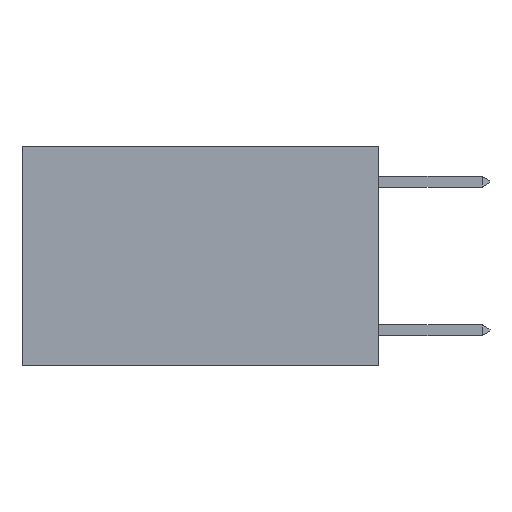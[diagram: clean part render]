
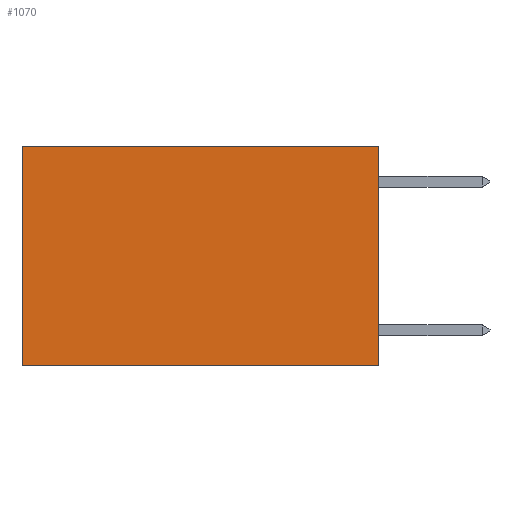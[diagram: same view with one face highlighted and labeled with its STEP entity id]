
A CAD part, left-side view. The second image highlights one B-rep face of the part: STEP entity #1070.
In plain terms, the highlighted planar face has unit normal (-1, 0, 0).
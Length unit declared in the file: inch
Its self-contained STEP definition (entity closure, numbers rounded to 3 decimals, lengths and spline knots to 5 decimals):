
#16 = VECTOR ( 'NONE', #1079, 39.37008 ) ;
#776 = AXIS2_PLACEMENT_3D ( 'NONE', #7842, #1541, #2116 ) ;
#898 = VERTEX_POINT ( 'NONE', #2107 ) ;
#1070 = ADVANCED_FACE ( 'NONE', ( #6622 ), #2194, .F. ) ;
#1079 = DIRECTION ( 'NONE',  ( 0., 1., 0. ) ) ;
#1117 = CARTESIAN_POINT ( 'NONE',  ( 0.2625, 0., 0. ) ) ;
#1541 = DIRECTION ( 'NONE',  ( 1., 0., 0. ) ) ;
#1621 = VERTEX_POINT ( 'NONE', #4800 ) ;
#1690 = VECTOR ( 'NONE', #4601, 39.37008 ) ;
#1726 = VECTOR ( 'NONE', #1788, 39.37008 ) ;
#1788 = DIRECTION ( 'NONE',  ( 0., 1., 0. ) ) ;
#2107 = CARTESIAN_POINT ( 'NONE',  ( 0.2625, 0., -0.37 ) ) ;
#2116 = DIRECTION ( 'NONE',  ( 0., 0., -1. ) ) ;
#2120 = LINE ( 'NONE', #5895, #4233 ) ;
#2194 = PLANE ( 'NONE',  #776 ) ;
#2446 = LINE ( 'NONE', #1117, #1690 ) ;
#2507 = DIRECTION ( 'NONE',  ( 0., 0., -1. ) ) ;
#2622 = ORIENTED_EDGE ( 'NONE', *, *, #3483, .T. ) ;
#3118 = CARTESIAN_POINT ( 'NONE',  ( 0.2625, 0., -0.37 ) ) ;
#3483 = EDGE_CURVE ( 'NONE', #6620, #1621, #2120, .T. ) ;
#3484 = CARTESIAN_POINT ( 'NONE',  ( 0.2625, 0., 0. ) ) ;
#4233 = VECTOR ( 'NONE', #2507, 39.37008 ) ;
#4429 = VERTEX_POINT ( 'NONE', #3484 ) ;
#4576 = EDGE_LOOP ( 'NONE', ( #2622, #8016, #7626, #7873 ) ) ;
#4601 = DIRECTION ( 'NONE',  ( 0., 0., -1. ) ) ;
#4800 = CARTESIAN_POINT ( 'NONE',  ( 0.2625, 0.6, -0.37 ) ) ;
#5773 = EDGE_CURVE ( 'NONE', #4429, #6620, #6756, .T. ) ;
#5895 = CARTESIAN_POINT ( 'NONE',  ( 0.2625, 0.6, 0. ) ) ;
#5929 = LINE ( 'NONE', #3118, #1726 ) ;
#6113 = CARTESIAN_POINT ( 'NONE',  ( 0.2625, 0., 0. ) ) ;
#6620 = VERTEX_POINT ( 'NONE', #8460 ) ;
#6622 = FACE_OUTER_BOUND ( 'NONE', #4576, .T. ) ;
#6685 = EDGE_CURVE ( 'NONE', #898, #1621, #5929, .T. ) ;
#6756 = LINE ( 'NONE', #6113, #16 ) ;
#7626 = ORIENTED_EDGE ( 'NONE', *, *, #8840, .F. ) ;
#7842 = CARTESIAN_POINT ( 'NONE',  ( 0.2625, 0., 0. ) ) ;
#7873 = ORIENTED_EDGE ( 'NONE', *, *, #5773, .T. ) ;
#8016 = ORIENTED_EDGE ( 'NONE', *, *, #6685, .F. ) ;
#8460 = CARTESIAN_POINT ( 'NONE',  ( 0.2625, 0.6, 0. ) ) ;
#8840 = EDGE_CURVE ( 'NONE', #4429, #898, #2446, .T. ) ;
